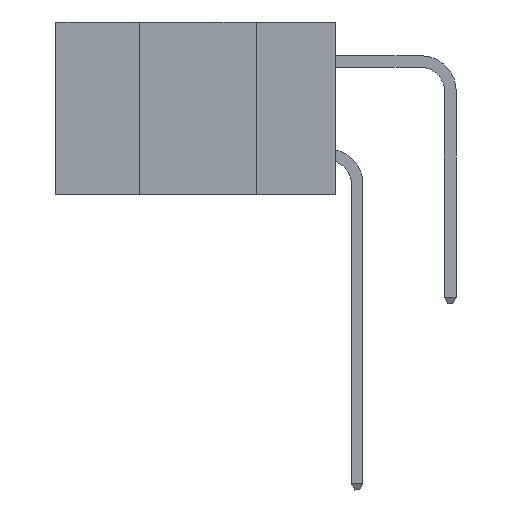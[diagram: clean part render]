
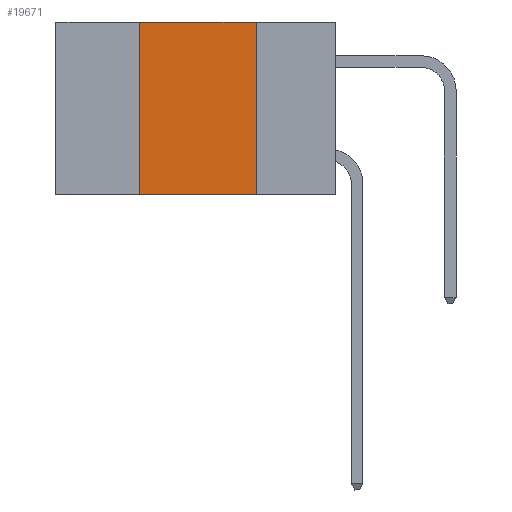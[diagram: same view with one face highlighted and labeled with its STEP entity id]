
A CAD part, left-side view. The second image highlights one B-rep face of the part: STEP entity #19671.
In plain terms, the highlighted planar face has unit normal (-1, 0, 0).
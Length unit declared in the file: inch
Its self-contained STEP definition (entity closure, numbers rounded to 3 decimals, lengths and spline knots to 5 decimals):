
#34 = EDGE_LOOP ( 'NONE', ( #2235, #16624, #28073, #26562 ) ) ;
#281 = EDGE_CURVE ( 'NONE', #25895, #14558, #9358, .T. ) ;
#715 = CARTESIAN_POINT ( 'NONE',  ( 0., 0.6, 0. ) ) ;
#1468 = LINE ( 'NONE', #19978, #6134 ) ;
#2003 = LINE ( 'NONE', #11567, #16770 ) ;
#2235 = ORIENTED_EDGE ( 'NONE', *, *, #281, .F. ) ;
#3122 = EDGE_CURVE ( 'NONE', #18587, #14558, #1468, .T. ) ;
#3596 = VECTOR ( 'NONE', #13068, 39.37008 ) ;
#4662 = EDGE_CURVE ( 'NONE', #19412, #25895, #24593, .T. ) ;
#6134 = VECTOR ( 'NONE', #26508, 39.37008 ) ;
#6350 = CARTESIAN_POINT ( 'NONE',  ( 0., 0.42, 0. ) ) ;
#7104 = DIRECTION ( 'NONE',  ( 0., 0., -1. ) ) ;
#7727 = FACE_OUTER_BOUND ( 'NONE', #34, .T. ) ;
#9358 = LINE ( 'NONE', #27871, #14761 ) ;
#11161 = AXIS2_PLACEMENT_3D ( 'NONE', #715, #21358, #21653 ) ;
#11567 = CARTESIAN_POINT ( 'NONE',  ( 0., 0.42, 0. ) ) ;
#12010 = CARTESIAN_POINT ( 'NONE',  ( 0., 0.42, -0.37 ) ) ;
#12583 = CARTESIAN_POINT ( 'NONE',  ( 0., 0.17, 0. ) ) ;
#13068 = DIRECTION ( 'NONE',  ( 0., -1., 0. ) ) ;
#14558 = VERTEX_POINT ( 'NONE', #20295 ) ;
#14761 = VECTOR ( 'NONE', #7104, 39.37008 ) ;
#16624 = ORIENTED_EDGE ( 'NONE', *, *, #4662, .F. ) ;
#16770 = VECTOR ( 'NONE', #20822, 39.37008 ) ;
#18587 = VERTEX_POINT ( 'NONE', #12010 ) ;
#19412 = VERTEX_POINT ( 'NONE', #6350 ) ;
#19671 = ADVANCED_FACE ( 'NONE', ( #7727 ), #28032, .F. ) ;
#19978 = CARTESIAN_POINT ( 'NONE',  ( 0., 0.6, -0.37 ) ) ;
#20295 = CARTESIAN_POINT ( 'NONE',  ( 0., 0.17, -0.37 ) ) ;
#20338 = CARTESIAN_POINT ( 'NONE',  ( 0., 0.6, 0. ) ) ;
#20822 = DIRECTION ( 'NONE',  ( 0., 0., 1. ) ) ;
#21358 = DIRECTION ( 'NONE',  ( 1., 0., 0. ) ) ;
#21653 = DIRECTION ( 'NONE',  ( 0., 0., -1. ) ) ;
#24593 = LINE ( 'NONE', #20338, #3596 ) ;
#25263 = EDGE_CURVE ( 'NONE', #18587, #19412, #2003, .T. ) ;
#25895 = VERTEX_POINT ( 'NONE', #12583 ) ;
#26508 = DIRECTION ( 'NONE',  ( 0., -1., 0. ) ) ;
#26562 = ORIENTED_EDGE ( 'NONE', *, *, #3122, .T. ) ;
#27871 = CARTESIAN_POINT ( 'NONE',  ( 0., 0.17, 0. ) ) ;
#28032 = PLANE ( 'NONE',  #11161 ) ;
#28073 = ORIENTED_EDGE ( 'NONE', *, *, #25263, .F. ) ;
